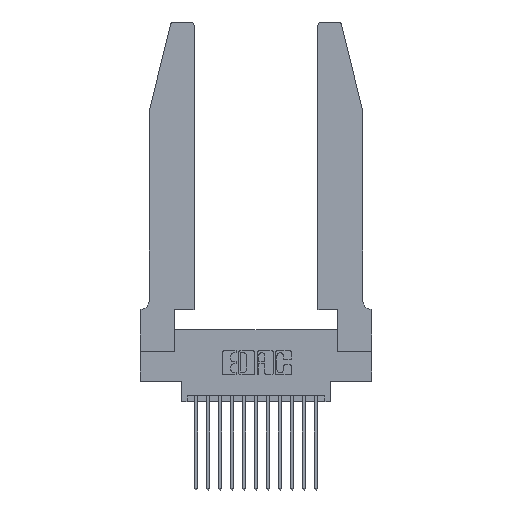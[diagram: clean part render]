
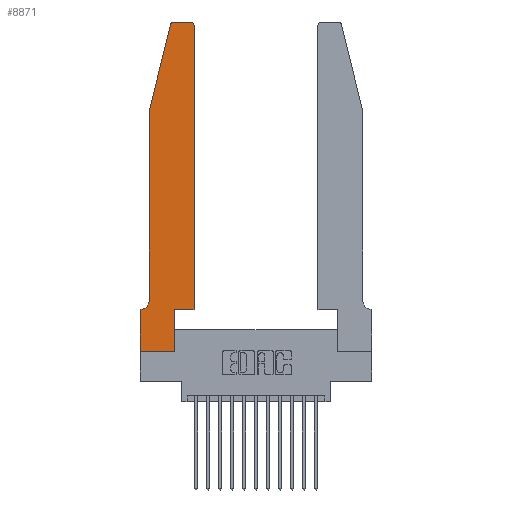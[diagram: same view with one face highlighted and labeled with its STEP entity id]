
A CAD part, top view. The second image highlights one B-rep face of the part: STEP entity #8871.
In plain terms, the highlighted planar face has unit normal (0, 0, 1).
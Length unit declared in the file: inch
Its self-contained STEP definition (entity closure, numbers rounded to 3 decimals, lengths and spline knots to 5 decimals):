
#323 = VERTEX_POINT ( 'NONE', #7245 ) ;
#398 = VECTOR ( 'NONE', #1914, 39.37008 ) ;
#523 = VERTEX_POINT ( 'NONE', #3846 ) ;
#745 = ORIENTED_EDGE ( 'NONE', *, *, #9212, .T. ) ;
#784 = EDGE_LOOP ( 'NONE', ( #745, #11922, #15778, #9133, #5835, #9566, #13171, #17004, #3001, #3453, #7188, #14404 ) ) ;
#826 = CARTESIAN_POINT ( 'NONE',  ( 0.0755, 2., 0.37 ) ) ;
#955 = DIRECTION ( 'NONE',  ( 0., 1., 0. ) ) ;
#1121 = CARTESIAN_POINT ( 'NONE',  ( 0.4205, 2.72, 0.37 ) ) ;
#1179 = VECTOR ( 'NONE', #17718, 39.37008 ) ;
#1636 = LINE ( 'NONE', #12532, #1179 ) ;
#1914 = DIRECTION ( 'NONE',  ( 1., 0., 0. ) ) ;
#2209 = LINE ( 'NONE', #3390, #12869 ) ;
#2226 = VECTOR ( 'NONE', #17295, 39.37008 ) ;
#2553 = DIRECTION ( 'NONE',  ( 1., 0., 0. ) ) ;
#2754 = DIRECTION ( 'NONE',  ( 0., 0., 1. ) ) ;
#2811 = LINE ( 'NONE', #14961, #9831 ) ;
#2998 = VERTEX_POINT ( 'NONE', #6287 ) ;
#3001 = ORIENTED_EDGE ( 'NONE', *, *, #13836, .T. ) ;
#3153 = CARTESIAN_POINT ( 'NONE',  ( 0.284, 2.75, 0.37 ) ) ;
#3191 = AXIS2_PLACEMENT_3D ( 'NONE', #1121, #10948, #2553 ) ;
#3349 = CIRCLE ( 'NONE', #15434, 0.07 ) ;
#3390 = CARTESIAN_POINT ( 'NONE',  ( 0.0755, 2., 0.37 ) ) ;
#3425 = VERTEX_POINT ( 'NONE', #12436 ) ;
#3453 = ORIENTED_EDGE ( 'NONE', *, *, #7567, .T. ) ;
#3770 = LINE ( 'NONE', #13022, #17706 ) ;
#3846 = CARTESIAN_POINT ( 'NONE',  ( 0.2865, 0., 0.37 ) ) ;
#4147 = VERTEX_POINT ( 'NONE', #826 ) ;
#4391 = DIRECTION ( 'NONE',  ( 0., 0., 1. ) ) ;
#4421 = CIRCLE ( 'NONE', #12004, 0.03 ) ;
#4804 = DIRECTION ( 'NONE',  ( 0., -1., 0. ) ) ;
#4868 = LINE ( 'NONE', #5545, #15312 ) ;
#5191 = CARTESIAN_POINT ( 'NONE',  ( 0.0055, 0.42, 0.37 ) ) ;
#5545 = CARTESIAN_POINT ( 'NONE',  ( 0.0755, 2., 0.37 ) ) ;
#5771 = CARTESIAN_POINT ( 'NONE',  ( 0.0755, 0.35, 0.37 ) ) ;
#5835 = ORIENTED_EDGE ( 'NONE', *, *, #14424, .T. ) ;
#6068 = CARTESIAN_POINT ( 'NONE',  ( 0.0055, 0.35, 0.37 ) ) ;
#6287 = CARTESIAN_POINT ( 'NONE',  ( 0.2865, 0.35, 0.37 ) ) ;
#6570 = CARTESIAN_POINT ( 'NONE',  ( 0.2865, 0.35, 0.37 ) ) ;
#6613 = DIRECTION ( 'NONE',  ( -1., 0., 0. ) ) ;
#6942 = CARTESIAN_POINT ( 'NONE',  ( 0., 0.35, 0.37 ) ) ;
#7188 = ORIENTED_EDGE ( 'NONE', *, *, #17418, .T. ) ;
#7245 = CARTESIAN_POINT ( 'NONE',  ( 0.4505, 0.35, 0.37 ) ) ;
#7290 = VERTEX_POINT ( 'NONE', #7697 ) ;
#7553 = FACE_OUTER_BOUND ( 'NONE', #784, .T. ) ;
#7567 = EDGE_CURVE ( 'NONE', #2998, #323, #1636, .T. ) ;
#7674 = LINE ( 'NONE', #5771, #10919 ) ;
#7697 = CARTESIAN_POINT ( 'NONE',  ( 0.0755, 0.42, 0.37 ) ) ;
#8871 = ADVANCED_FACE ( 'NONE', ( #7553 ), #11141, .T. ) ;
#9133 = ORIENTED_EDGE ( 'NONE', *, *, #15255, .T. ) ;
#9212 = EDGE_CURVE ( 'NONE', #3425, #13605, #15894, .T. ) ;
#9495 = VERTEX_POINT ( 'NONE', #15328 ) ;
#9566 = ORIENTED_EDGE ( 'NONE', *, *, #17589, .T. ) ;
#9639 = DIRECTION ( 'NONE',  ( 0., 1., 0. ) ) ;
#9672 = EDGE_CURVE ( 'NONE', #16406, #4147, #2209, .T. ) ;
#9831 = VECTOR ( 'NONE', #9639, 39.37008 ) ;
#10762 = EDGE_CURVE ( 'NONE', #13605, #16406, #4421, .T. ) ;
#10919 = VECTOR ( 'NONE', #15282, 39.37008 ) ;
#10948 = DIRECTION ( 'NONE',  ( 0., 0., 1. ) ) ;
#11141 = PLANE ( 'NONE',  #13989 ) ;
#11689 = CARTESIAN_POINT ( 'NONE',  ( 0., 0., 0.37 ) ) ;
#11916 = LINE ( 'NONE', #6570, #13779 ) ;
#11922 = ORIENTED_EDGE ( 'NONE', *, *, #10762, .T. ) ;
#12004 = AXIS2_PLACEMENT_3D ( 'NONE', #12686, #4391, #14008 ) ;
#12427 = CARTESIAN_POINT ( 'NONE',  ( 0., 0., 0.37 ) ) ;
#12436 = CARTESIAN_POINT ( 'NONE',  ( 0.4205, 2.75, 0.37 ) ) ;
#12452 = DIRECTION ( 'NONE',  ( 0., -1., 0. ) ) ;
#12487 = DIRECTION ( 'NONE',  ( 1., 0., 0. ) ) ;
#12532 = CARTESIAN_POINT ( 'NONE',  ( 0.4505, 0.35, 0.37 ) ) ;
#12686 = CARTESIAN_POINT ( 'NONE',  ( 0.284, 2.72, 0.37 ) ) ;
#12869 = VECTOR ( 'NONE', #13057, 39.37008 ) ;
#13022 = CARTESIAN_POINT ( 'NONE',  ( 0., 0., 0.37 ) ) ;
#13057 = DIRECTION ( 'NONE',  ( -0.239, -0.971, 0. ) ) ;
#13083 = CIRCLE ( 'NONE', #3191, 0.03 ) ;
#13171 = ORIENTED_EDGE ( 'NONE', *, *, #15575, .T. ) ;
#13605 = VERTEX_POINT ( 'NONE', #3153 ) ;
#13779 = VECTOR ( 'NONE', #955, 39.37008 ) ;
#13836 = EDGE_CURVE ( 'NONE', #523, #2998, #11916, .T. ) ;
#13960 = VERTEX_POINT ( 'NONE', #12427 ) ;
#13989 = AXIS2_PLACEMENT_3D ( 'NONE', #6942, #2754, #12487 ) ;
#14008 = DIRECTION ( 'NONE',  ( 1., 0., 0. ) ) ;
#14404 = ORIENTED_EDGE ( 'NONE', *, *, #14492, .T. ) ;
#14424 = EDGE_CURVE ( 'NONE', #7290, #16114, #3349, .T. ) ;
#14492 = EDGE_CURVE ( 'NONE', #9495, #3425, #13083, .T. ) ;
#14735 = CARTESIAN_POINT ( 'NONE',  ( 0.2605, 2.75, 0.37 ) ) ;
#14766 = DIRECTION ( 'NONE',  ( 0., 0., -1. ) ) ;
#14961 = CARTESIAN_POINT ( 'NONE',  ( 0.4505, 0.35, 0.37 ) ) ;
#15116 = LINE ( 'NONE', #11689, #398 ) ;
#15255 = EDGE_CURVE ( 'NONE', #4147, #7290, #4868, .T. ) ;
#15282 = DIRECTION ( 'NONE',  ( -1., 0., 0. ) ) ;
#15312 = VECTOR ( 'NONE', #12452, 39.37008 ) ;
#15328 = CARTESIAN_POINT ( 'NONE',  ( 0.4505, 2.72, 0.37 ) ) ;
#15434 = AXIS2_PLACEMENT_3D ( 'NONE', #5191, #14766, #6613 ) ;
#15551 = EDGE_CURVE ( 'NONE', #13960, #523, #15116, .T. ) ;
#15575 = EDGE_CURVE ( 'NONE', #16513, #13960, #3770, .T. ) ;
#15778 = ORIENTED_EDGE ( 'NONE', *, *, #9672, .T. ) ;
#15894 = LINE ( 'NONE', #14735, #2226 ) ;
#16114 = VERTEX_POINT ( 'NONE', #6068 ) ;
#16406 = VERTEX_POINT ( 'NONE', #17387 ) ;
#16513 = VERTEX_POINT ( 'NONE', #16531 ) ;
#16531 = CARTESIAN_POINT ( 'NONE',  ( 0., 0.35, 0.37 ) ) ;
#17004 = ORIENTED_EDGE ( 'NONE', *, *, #15551, .T. ) ;
#17295 = DIRECTION ( 'NONE',  ( -1., 0., 0. ) ) ;
#17387 = CARTESIAN_POINT ( 'NONE',  ( 0.25487, 2.72718, 0.37 ) ) ;
#17418 = EDGE_CURVE ( 'NONE', #323, #9495, #2811, .T. ) ;
#17589 = EDGE_CURVE ( 'NONE', #16114, #16513, #7674, .T. ) ;
#17706 = VECTOR ( 'NONE', #4804, 39.37008 ) ;
#17718 = DIRECTION ( 'NONE',  ( 1., 0., 0. ) ) ;
